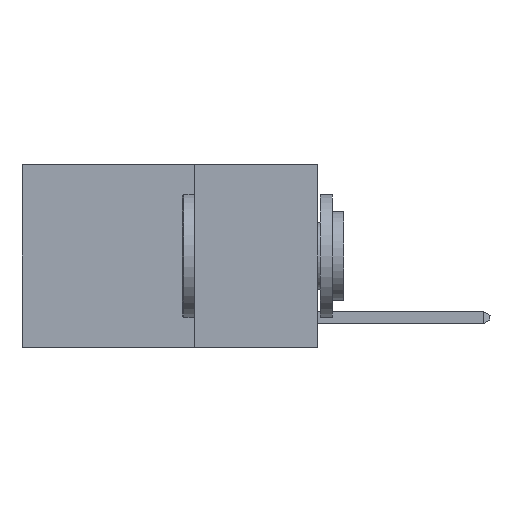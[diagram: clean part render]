
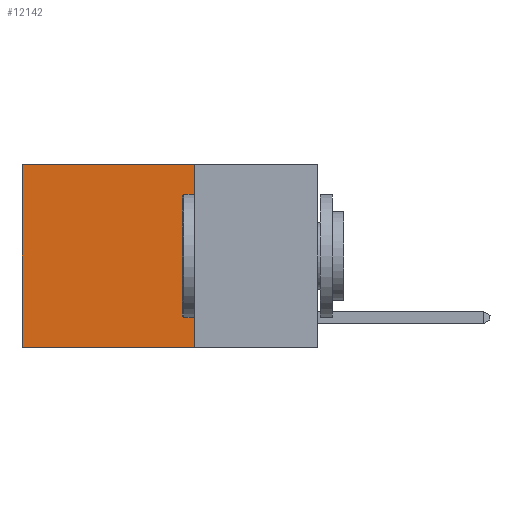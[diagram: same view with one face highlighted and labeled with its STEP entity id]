
A CAD part, left-side view. The second image highlights one B-rep face of the part: STEP entity #12142.
In plain terms, the highlighted planar face has unit normal (-1, 0, 0).
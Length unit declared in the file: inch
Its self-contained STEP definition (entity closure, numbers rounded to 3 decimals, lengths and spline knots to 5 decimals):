
#95 = EDGE_CURVE ( 'NONE', #5966, #16044, #14713, .T. ) ;
#1020 = LINE ( 'NONE', #1143, #7203 ) ;
#1104 = EDGE_CURVE ( 'NONE', #14304, #1687, #15846, .T. ) ;
#1143 = CARTESIAN_POINT ( 'NONE',  ( 0.2625, 0.25, -0.37 ) ) ;
#1687 = VERTEX_POINT ( 'NONE', #16486 ) ;
#2084 = VECTOR ( 'NONE', #23713, 39.37008 ) ;
#2112 = DIRECTION ( 'NONE',  ( 1., 0., 0. ) ) ;
#2358 = PLANE ( 'NONE',  #20453 ) ;
#2481 = DIRECTION ( 'NONE',  ( 0., 0., -1. ) ) ;
#3663 = LINE ( 'NONE', #11203, #14595 ) ;
#5407 = DIRECTION ( 'NONE',  ( 0., 0., -1. ) ) ;
#5966 = VERTEX_POINT ( 'NONE', #21083 ) ;
#6373 = FACE_OUTER_BOUND ( 'NONE', #16635, .T. ) ;
#7203 = VECTOR ( 'NONE', #14245, 39.37008 ) ;
#7517 = CARTESIAN_POINT ( 'NONE',  ( 0.2625, 0.25, 0. ) ) ;
#7549 = DIRECTION ( 'NONE',  ( 0., 1., 0. ) ) ;
#10984 = ORIENTED_EDGE ( 'NONE', *, *, #15061, .F. ) ;
#11203 = CARTESIAN_POINT ( 'NONE',  ( 0.2625, 0.25, 0. ) ) ;
#11763 = ORIENTED_EDGE ( 'NONE', *, *, #14405, .T. ) ;
#12142 = ADVANCED_FACE ( 'NONE', ( #6373 ), #2358, .F. ) ;
#12601 = ORIENTED_EDGE ( 'NONE', *, *, #95, .F. ) ;
#12618 = CARTESIAN_POINT ( 'NONE',  ( 0.2625, 0.6, 0. ) ) ;
#14245 = DIRECTION ( 'NONE',  ( 0., 1., 0. ) ) ;
#14304 = VERTEX_POINT ( 'NONE', #21233 ) ;
#14405 = EDGE_CURVE ( 'NONE', #5966, #14304, #3663, .T. ) ;
#14595 = VECTOR ( 'NONE', #7549, 39.37008 ) ;
#14713 = LINE ( 'NONE', #7517, #21556 ) ;
#15061 = EDGE_CURVE ( 'NONE', #16044, #1687, #1020, .T. ) ;
#15846 = LINE ( 'NONE', #12618, #2084 ) ;
#16044 = VERTEX_POINT ( 'NONE', #22778 ) ;
#16486 = CARTESIAN_POINT ( 'NONE',  ( 0.2625, 0.6, -0.37 ) ) ;
#16635 = EDGE_LOOP ( 'NONE', ( #19223, #10984, #12601, #11763 ) ) ;
#19223 = ORIENTED_EDGE ( 'NONE', *, *, #1104, .T. ) ;
#19608 = CARTESIAN_POINT ( 'NONE',  ( 0.2625, 0.25, 0. ) ) ;
#20453 = AXIS2_PLACEMENT_3D ( 'NONE', #19608, #2112, #2481 ) ;
#21083 = CARTESIAN_POINT ( 'NONE',  ( 0.2625, 0.25, 0. ) ) ;
#21233 = CARTESIAN_POINT ( 'NONE',  ( 0.2625, 0.6, 0. ) ) ;
#21556 = VECTOR ( 'NONE', #5407, 39.37008 ) ;
#22778 = CARTESIAN_POINT ( 'NONE',  ( 0.2625, 0.25, -0.37 ) ) ;
#23713 = DIRECTION ( 'NONE',  ( 0., 0., -1. ) ) ;
